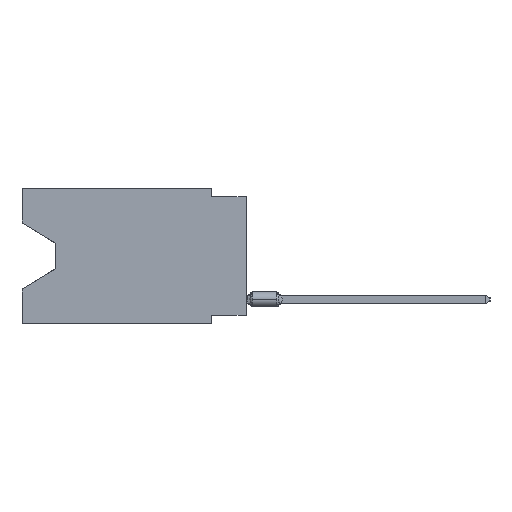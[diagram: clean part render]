
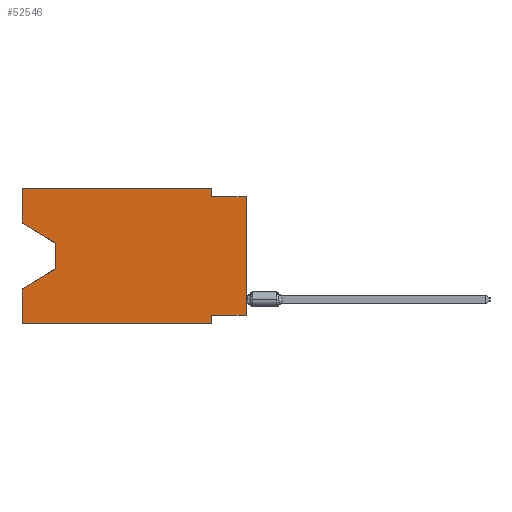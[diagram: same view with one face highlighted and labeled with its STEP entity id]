
A CAD part, left-side view. The second image highlights one B-rep face of the part: STEP entity #52546.
In plain terms, the highlighted planar face has unit normal (-1, 0, 0).
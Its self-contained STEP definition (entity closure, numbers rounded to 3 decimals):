
#132 = LINE ( 'NONE', #19713, #51096 ) ;
#422 = LINE ( 'NONE', #29311, #62301 ) ;
#656 = CARTESIAN_POINT ( 'NONE',  ( 0., 13.97, -4.013 ) ) ;
#874 = CARTESIAN_POINT ( 'NONE',  ( 0., 13.97, -5.893 ) ) ;
#3740 = ORIENTED_EDGE ( 'NONE', *, *, #4860, .F. ) ;
#3807 = DIRECTION ( 'NONE',  ( 1., 0., 0. ) ) ;
#3827 = ORIENTED_EDGE ( 'NONE', *, *, #24298, .T. ) ;
#4141 = CARTESIAN_POINT ( 'NONE',  ( 0., 16.383, 0. ) ) ;
#4849 = LINE ( 'NONE', #656, #59069 ) ;
#4860 = EDGE_CURVE ( 'NONE', #39438, #45369, #11494, .T. ) ;
#5394 = VECTOR ( 'NONE', #18892, 1000. ) ;
#6302 = VERTEX_POINT ( 'NONE', #14006 ) ;
#7177 = EDGE_CURVE ( 'NONE', #62593, #38720, #44475, .T. ) ;
#8340 = EDGE_CURVE ( 'NONE', #6302, #60881, #37743, .T. ) ;
#8634 = EDGE_CURVE ( 'NONE', #63139, #56007, #47445, .T. ) ;
#9801 = LINE ( 'NONE', #29083, #63425 ) ;
#11494 = LINE ( 'NONE', #20492, #44838 ) ;
#12944 = LINE ( 'NONE', #41531, #20523 ) ;
#13001 = ORIENTED_EDGE ( 'NONE', *, *, #7177, .F. ) ;
#13100 = VECTOR ( 'NONE', #44385, 1000. ) ;
#13129 = CARTESIAN_POINT ( 'NONE',  ( 0., 16.383, 0. ) ) ;
#13372 = DIRECTION ( 'NONE',  ( 0., 0., 1. ) ) ;
#13463 = EDGE_LOOP ( 'NONE', ( #3827, #31619, #50655, #27951, #53363, #3740, #40305, #14719, #43205, #13001, #23370, #38479 ) ) ;
#14006 = CARTESIAN_POINT ( 'NONE',  ( 0., 0., -9.271 ) ) ;
#14593 = CARTESIAN_POINT ( 'NONE',  ( 0., 16.383, -7.36 ) ) ;
#14719 = ORIENTED_EDGE ( 'NONE', *, *, #8340, .T. ) ;
#16984 = VECTOR ( 'NONE', #25021, 1000. ) ;
#17120 = DIRECTION ( 'NONE',  ( 0., -1., 0. ) ) ;
#17243 = CARTESIAN_POINT ( 'NONE',  ( 0., 0., -0.635 ) ) ;
#17524 = VERTEX_POINT ( 'NONE', #49802 ) ;
#17695 = CARTESIAN_POINT ( 'NONE',  ( 0., 2.54, -9.271 ) ) ;
#17908 = CARTESIAN_POINT ( 'NONE',  ( 0., 2.54, -9.906 ) ) ;
#18248 = DIRECTION ( 'NONE',  ( 0., 0., -1. ) ) ;
#18892 = DIRECTION ( 'NONE',  ( 0., 0., 1. ) ) ;
#19212 = PLANE ( 'NONE',  #43877 ) ;
#19560 = FACE_OUTER_BOUND ( 'NONE', #13463, .T. ) ;
#19713 = CARTESIAN_POINT ( 'NONE',  ( 0., 16.383, -2.546 ) ) ;
#19783 = DIRECTION ( 'NONE',  ( 0., 0., -1. ) ) ;
#20464 = EDGE_CURVE ( 'NONE', #6302, #39438, #60316, .T. ) ;
#20492 = CARTESIAN_POINT ( 'NONE',  ( 0., 2.54, -9.906 ) ) ;
#20523 = VECTOR ( 'NONE', #17120, 1000. ) ;
#21147 = CARTESIAN_POINT ( 'NONE',  ( 0., 16.383, -9.906 ) ) ;
#21630 = EDGE_CURVE ( 'NONE', #55168, #45369, #58837, .T. ) ;
#23370 = ORIENTED_EDGE ( 'NONE', *, *, #26607, .F. ) ;
#24298 = EDGE_CURVE ( 'NONE', #63139, #17524, #132, .T. ) ;
#24455 = CARTESIAN_POINT ( 'NONE',  ( 0., 16.383, -2.546 ) ) ;
#24660 = EDGE_CURVE ( 'NONE', #17524, #45582, #4849, .T. ) ;
#24840 = DIRECTION ( 'NONE',  ( 0., -0.855, -0.519 ) ) ;
#25021 = DIRECTION ( 'NONE',  ( 0., 1., 0. ) ) ;
#26607 = EDGE_CURVE ( 'NONE', #56007, #62593, #422, .T. ) ;
#27178 = EDGE_CURVE ( 'NONE', #45582, #30946, #9801, .T. ) ;
#27750 = DIRECTION ( 'NONE',  ( 0., 0., 1. ) ) ;
#27951 = ORIENTED_EDGE ( 'NONE', *, *, #54566, .F. ) ;
#28713 = LINE ( 'NONE', #48605, #42996 ) ;
#29083 = CARTESIAN_POINT ( 'NONE',  ( 0., 13.97, -5.893 ) ) ;
#29311 = CARTESIAN_POINT ( 'NONE',  ( 0., 16.383, 0. ) ) ;
#30946 = VERTEX_POINT ( 'NONE', #14593 ) ;
#31361 = DIRECTION ( 'NONE',  ( 0., 0., -1. ) ) ;
#31619 = ORIENTED_EDGE ( 'NONE', *, *, #24660, .T. ) ;
#34444 = DIRECTION ( 'NONE',  ( 0., -1., 0. ) ) ;
#34818 = VECTOR ( 'NONE', #19783, 1000. ) ;
#35258 = DIRECTION ( 'NONE',  ( 0., 0., -1. ) ) ;
#37743 = LINE ( 'NONE', #57337, #54394 ) ;
#38479 = ORIENTED_EDGE ( 'NONE', *, *, #8634, .F. ) ;
#38695 = DIRECTION ( 'NONE',  ( 0., 0.855, -0.519 ) ) ;
#38720 = VERTEX_POINT ( 'NONE', #48945 ) ;
#39095 = EDGE_CURVE ( 'NONE', #38720, #60881, #12944, .T. ) ;
#39438 = VERTEX_POINT ( 'NONE', #17695 ) ;
#40305 = ORIENTED_EDGE ( 'NONE', *, *, #20464, .F. ) ;
#41531 = CARTESIAN_POINT ( 'NONE',  ( 0., 0., -0.635 ) ) ;
#42996 = VECTOR ( 'NONE', #27750, 1000. ) ;
#43205 = ORIENTED_EDGE ( 'NONE', *, *, #39095, .F. ) ;
#43877 = AXIS2_PLACEMENT_3D ( 'NONE', #48739, #3807, #18248 ) ;
#44385 = DIRECTION ( 'NONE',  ( 0., -1., 0. ) ) ;
#44475 = LINE ( 'NONE', #63091, #34818 ) ;
#44838 = VECTOR ( 'NONE', #35258, 1000. ) ;
#45369 = VERTEX_POINT ( 'NONE', #17908 ) ;
#45582 = VERTEX_POINT ( 'NONE', #874 ) ;
#47445 = LINE ( 'NONE', #4141, #5394 ) ;
#48605 = CARTESIAN_POINT ( 'NONE',  ( 0., 16.383, 0. ) ) ;
#48739 = CARTESIAN_POINT ( 'NONE',  ( 0., 16.383, 0. ) ) ;
#48945 = CARTESIAN_POINT ( 'NONE',  ( 0., 2.54, -0.635 ) ) ;
#49802 = CARTESIAN_POINT ( 'NONE',  ( 0., 13.97, -4.013 ) ) ;
#50369 = CARTESIAN_POINT ( 'NONE',  ( 0., 0., -9.271 ) ) ;
#50655 = ORIENTED_EDGE ( 'NONE', *, *, #27178, .T. ) ;
#51096 = VECTOR ( 'NONE', #24840, 1000. ) ;
#52123 = CARTESIAN_POINT ( 'NONE',  ( 0., 16.383, -9.906 ) ) ;
#52546 = ADVANCED_FACE ( 'NONE', ( #19560 ), #19212, .F. ) ;
#53363 = ORIENTED_EDGE ( 'NONE', *, *, #21630, .T. ) ;
#54394 = VECTOR ( 'NONE', #13372, 1000. ) ;
#54566 = EDGE_CURVE ( 'NONE', #55168, #30946, #28713, .T. ) ;
#55168 = VERTEX_POINT ( 'NONE', #52123 ) ;
#56007 = VERTEX_POINT ( 'NONE', #13129 ) ;
#57337 = CARTESIAN_POINT ( 'NONE',  ( 0., 0., 0. ) ) ;
#57613 = CARTESIAN_POINT ( 'NONE',  ( 0., 2.54, 0. ) ) ;
#58837 = LINE ( 'NONE', #21147, #13100 ) ;
#59069 = VECTOR ( 'NONE', #31361, 1000. ) ;
#60316 = LINE ( 'NONE', #50369, #16984 ) ;
#60881 = VERTEX_POINT ( 'NONE', #17243 ) ;
#62301 = VECTOR ( 'NONE', #34444, 1000. ) ;
#62593 = VERTEX_POINT ( 'NONE', #57613 ) ;
#63091 = CARTESIAN_POINT ( 'NONE',  ( 0., 2.54, 0. ) ) ;
#63139 = VERTEX_POINT ( 'NONE', #24455 ) ;
#63425 = VECTOR ( 'NONE', #38695, 1000. ) ;
